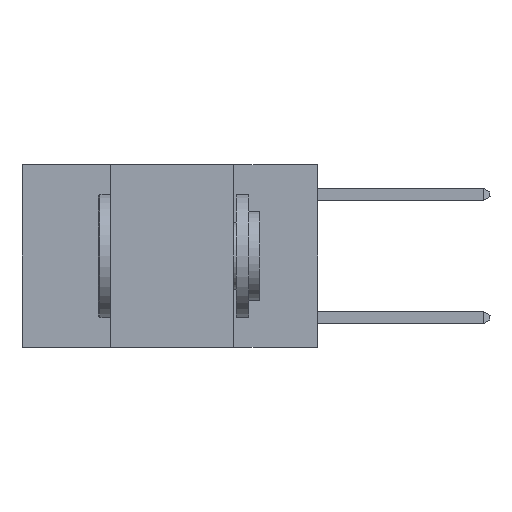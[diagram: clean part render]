
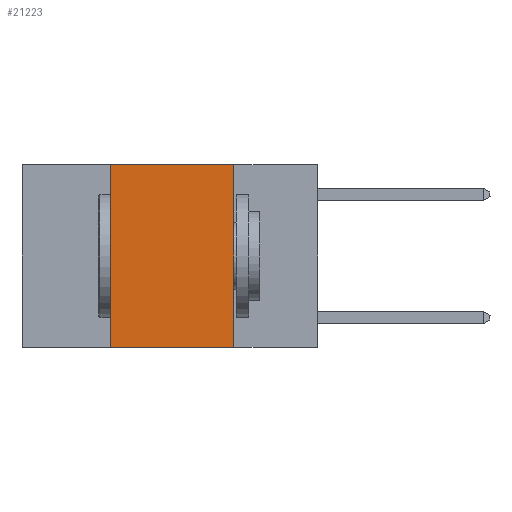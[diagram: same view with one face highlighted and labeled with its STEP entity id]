
A CAD part, left-side view. The second image highlights one B-rep face of the part: STEP entity #21223.
In plain terms, the highlighted planar face has unit normal (-1, 0, 0).
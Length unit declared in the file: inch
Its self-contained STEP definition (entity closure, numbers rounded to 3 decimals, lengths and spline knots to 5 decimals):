
#695 = VECTOR ( 'NONE', #14296, 39.37008 ) ;
#1761 = CARTESIAN_POINT ( 'NONE',  ( 0., 0.6, 0. ) ) ;
#3044 = VECTOR ( 'NONE', #24456, 39.37008 ) ;
#3639 = CARTESIAN_POINT ( 'NONE',  ( 0., 0.6, 0. ) ) ;
#3777 = ORIENTED_EDGE ( 'NONE', *, *, #21429, .T. ) ;
#6528 = ORIENTED_EDGE ( 'NONE', *, *, #16075, .F. ) ;
#6715 = AXIS2_PLACEMENT_3D ( 'NONE', #3639, #11195, #18904 ) ;
#6767 = LINE ( 'NONE', #14776, #695 ) ;
#7291 = EDGE_CURVE ( 'NONE', #16572, #7369, #6767, .T. ) ;
#7369 = VERTEX_POINT ( 'NONE', #11721 ) ;
#7775 = ORIENTED_EDGE ( 'NONE', *, *, #12877, .F. ) ;
#7866 = CARTESIAN_POINT ( 'NONE',  ( 0., 0.42, 0. ) ) ;
#9109 = FACE_OUTER_BOUND ( 'NONE', #17804, .T. ) ;
#11152 = ORIENTED_EDGE ( 'NONE', *, *, #7291, .F. ) ;
#11192 = LINE ( 'NONE', #1761, #21395 ) ;
#11195 = DIRECTION ( 'NONE',  ( 1., 0., 0. ) ) ;
#11721 = CARTESIAN_POINT ( 'NONE',  ( 0., 0.17, -0.37 ) ) ;
#12877 = EDGE_CURVE ( 'NONE', #22792, #16572, #11192, .T. ) ;
#13651 = DIRECTION ( 'NONE',  ( 0., -1., 0. ) ) ;
#14296 = DIRECTION ( 'NONE',  ( 0., 0., -1. ) ) ;
#14615 = CARTESIAN_POINT ( 'NONE',  ( 0., 0.42, 0. ) ) ;
#14771 = DIRECTION ( 'NONE',  ( 0., -1., 0. ) ) ;
#14776 = CARTESIAN_POINT ( 'NONE',  ( 0., 0.17, 0. ) ) ;
#15812 = VECTOR ( 'NONE', #13651, 39.37008 ) ;
#16075 = EDGE_CURVE ( 'NONE', #22490, #22792, #24086, .T. ) ;
#16401 = CARTESIAN_POINT ( 'NONE',  ( 0., 0.42, -0.37 ) ) ;
#16572 = VERTEX_POINT ( 'NONE', #22400 ) ;
#17804 = EDGE_LOOP ( 'NONE', ( #11152, #7775, #6528, #3777 ) ) ;
#18904 = DIRECTION ( 'NONE',  ( 0., 0., -1. ) ) ;
#19148 = CARTESIAN_POINT ( 'NONE',  ( 0., 0.6, -0.37 ) ) ;
#19270 = LINE ( 'NONE', #19148, #15812 ) ;
#20510 = PLANE ( 'NONE',  #6715 ) ;
#21223 = ADVANCED_FACE ( 'NONE', ( #9109 ), #20510, .F. ) ;
#21395 = VECTOR ( 'NONE', #14771, 39.37008 ) ;
#21429 = EDGE_CURVE ( 'NONE', #22490, #7369, #19270, .T. ) ;
#22400 = CARTESIAN_POINT ( 'NONE',  ( 0., 0.17, 0. ) ) ;
#22490 = VERTEX_POINT ( 'NONE', #16401 ) ;
#22792 = VERTEX_POINT ( 'NONE', #7866 ) ;
#24086 = LINE ( 'NONE', #14615, #3044 ) ;
#24456 = DIRECTION ( 'NONE',  ( 0., 0., 1. ) ) ;
